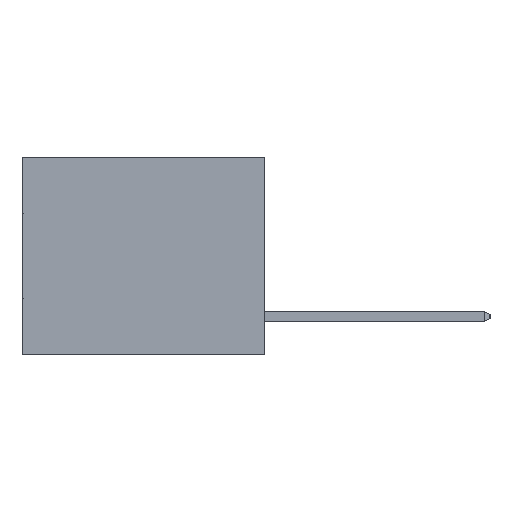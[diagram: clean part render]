
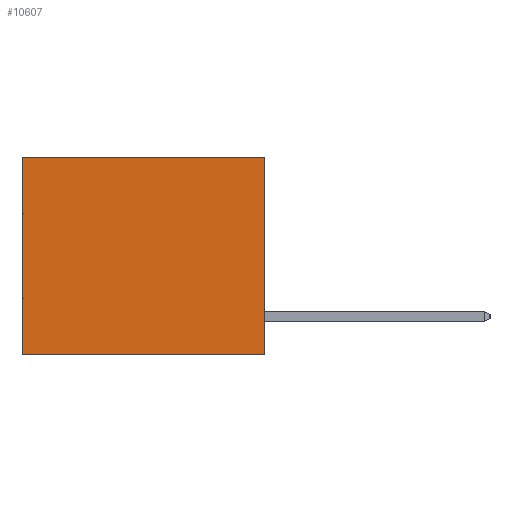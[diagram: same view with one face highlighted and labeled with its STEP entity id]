
A CAD part, left-side view. The second image highlights one B-rep face of the part: STEP entity #10607.
In plain terms, the highlighted planar face has unit normal (-1, 0, 0).
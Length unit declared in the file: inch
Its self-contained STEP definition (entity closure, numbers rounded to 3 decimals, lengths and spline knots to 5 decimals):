
#1852 = LINE ( 'NONE', #24939, #12840 ) ;
#3320 = EDGE_LOOP ( 'NONE', ( #29355, #31718, #10686, #10408 ) ) ;
#4337 = CARTESIAN_POINT ( 'NONE',  ( 0.3165, 0., -0.49 ) ) ;
#5017 = DIRECTION ( 'NONE',  ( 0., 1., 0. ) ) ;
#5733 = LINE ( 'NONE', #24931, #11594 ) ;
#6457 = CARTESIAN_POINT ( 'NONE',  ( 0.3165, 0.6, 0. ) ) ;
#6961 = VECTOR ( 'NONE', #31363, 39.37008 ) ;
#7723 = VERTEX_POINT ( 'NONE', #23890 ) ;
#10408 = ORIENTED_EDGE ( 'NONE', *, *, #28398, .T. ) ;
#10607 = ADVANCED_FACE ( 'NONE', ( #31764 ), #10971, .F. ) ;
#10686 = ORIENTED_EDGE ( 'NONE', *, *, #17231, .F. ) ;
#10971 = PLANE ( 'NONE',  #19349 ) ;
#11188 = CARTESIAN_POINT ( 'NONE',  ( 0.3165, 0., -0.49 ) ) ;
#11594 = VECTOR ( 'NONE', #29492, 39.37008 ) ;
#12840 = VECTOR ( 'NONE', #5017, 39.37008 ) ;
#17231 = EDGE_CURVE ( 'NONE', #18680, #20324, #25446, .T. ) ;
#18680 = VERTEX_POINT ( 'NONE', #31239 ) ;
#19349 = AXIS2_PLACEMENT_3D ( 'NONE', #11188, #28744, #26313 ) ;
#20266 = EDGE_CURVE ( 'NONE', #32408, #7723, #5733, .T. ) ;
#20324 = VERTEX_POINT ( 'NONE', #4337 ) ;
#23890 = CARTESIAN_POINT ( 'NONE',  ( 0.3165, 0.6, -0.49 ) ) ;
#24747 = VECTOR ( 'NONE', #32468, 39.37008 ) ;
#24931 = CARTESIAN_POINT ( 'NONE',  ( 0.3165, 0.6, -0.49 ) ) ;
#24939 = CARTESIAN_POINT ( 'NONE',  ( 0.3165, 0., 0. ) ) ;
#25446 = LINE ( 'NONE', #28934, #6961 ) ;
#26313 = DIRECTION ( 'NONE',  ( 0., 0., -1. ) ) ;
#27087 = EDGE_CURVE ( 'NONE', #20324, #7723, #31472, .T. ) ;
#28398 = EDGE_CURVE ( 'NONE', #18680, #32408, #1852, .T. ) ;
#28744 = DIRECTION ( 'NONE',  ( 1., 0., 0. ) ) ;
#28934 = CARTESIAN_POINT ( 'NONE',  ( 0.3165, 0., -0.49 ) ) ;
#29355 = ORIENTED_EDGE ( 'NONE', *, *, #20266, .T. ) ;
#29492 = DIRECTION ( 'NONE',  ( 0., 0., -1. ) ) ;
#31239 = CARTESIAN_POINT ( 'NONE',  ( 0.3165, 0., 0. ) ) ;
#31363 = DIRECTION ( 'NONE',  ( 0., 0., -1. ) ) ;
#31472 = LINE ( 'NONE', #32357, #24747 ) ;
#31718 = ORIENTED_EDGE ( 'NONE', *, *, #27087, .F. ) ;
#31764 = FACE_OUTER_BOUND ( 'NONE', #3320, .T. ) ;
#32357 = CARTESIAN_POINT ( 'NONE',  ( 0.3165, 0., -0.49 ) ) ;
#32408 = VERTEX_POINT ( 'NONE', #6457 ) ;
#32468 = DIRECTION ( 'NONE',  ( 0., 1., 0. ) ) ;
